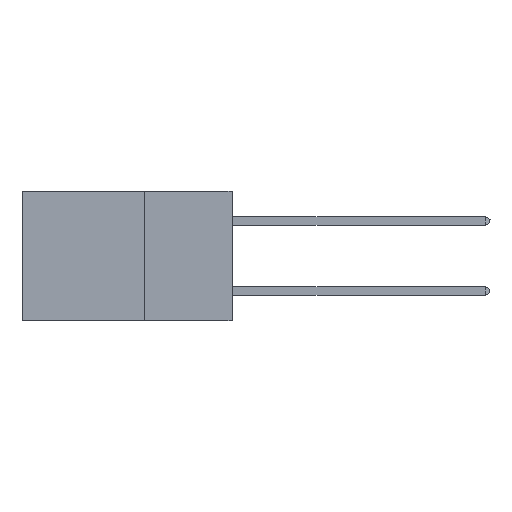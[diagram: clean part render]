
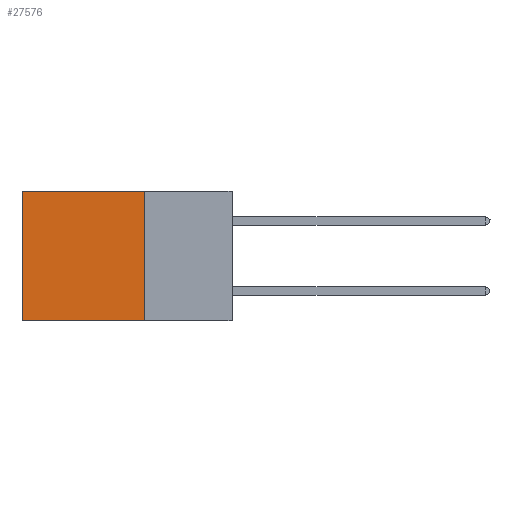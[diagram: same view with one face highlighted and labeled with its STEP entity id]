
A CAD part, left-side view. The second image highlights one B-rep face of the part: STEP entity #27576.
In plain terms, the highlighted planar face has unit normal (-1, 0, 0).
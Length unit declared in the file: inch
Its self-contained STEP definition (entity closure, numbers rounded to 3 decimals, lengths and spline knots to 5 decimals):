
#475 = ORIENTED_EDGE ( 'NONE', *, *, #20749, .F. ) ;
#2048 = VERTEX_POINT ( 'NONE', #22306 ) ;
#2935 = FACE_OUTER_BOUND ( 'NONE', #39956, .T. ) ;
#2964 = ORIENTED_EDGE ( 'NONE', *, *, #19915, .T. ) ;
#4848 = CARTESIAN_POINT ( 'NONE',  ( 0.2875, 0.25, -0.37 ) ) ;
#4908 = CARTESIAN_POINT ( 'NONE',  ( 0.2875, 0.25, 0. ) ) ;
#5237 = DIRECTION ( 'NONE',  ( 0., 0., -1. ) ) ;
#6970 = ORIENTED_EDGE ( 'NONE', *, *, #25599, .F. ) ;
#7284 = CARTESIAN_POINT ( 'NONE',  ( 0.2875, 0.25, 0. ) ) ;
#7676 = DIRECTION ( 'NONE',  ( 0., 1., 0. ) ) ;
#8285 = LINE ( 'NONE', #22041, #31286 ) ;
#8759 = LINE ( 'NONE', #9410, #9766 ) ;
#9410 = CARTESIAN_POINT ( 'NONE',  ( 0.2875, 0.25, 0. ) ) ;
#9766 = VECTOR ( 'NONE', #35423, 39.37008 ) ;
#9790 = VERTEX_POINT ( 'NONE', #36694 ) ;
#11019 = LINE ( 'NONE', #4908, #34777 ) ;
#15156 = VERTEX_POINT ( 'NONE', #33258 ) ;
#17466 = ORIENTED_EDGE ( 'NONE', *, *, #27463, .T. ) ;
#18236 = AXIS2_PLACEMENT_3D ( 'NONE', #39439, #33085, #42938 ) ;
#19915 = EDGE_CURVE ( 'NONE', #2048, #9790, #8285, .T. ) ;
#20749 = EDGE_CURVE ( 'NONE', #15156, #9790, #24489, .T. ) ;
#22041 = CARTESIAN_POINT ( 'NONE',  ( 0.2875, 0.6, 0. ) ) ;
#22306 = CARTESIAN_POINT ( 'NONE',  ( 0.2875, 0.6, 0. ) ) ;
#24489 = LINE ( 'NONE', #4848, #31104 ) ;
#25599 = EDGE_CURVE ( 'NONE', #35678, #15156, #8759, .T. ) ;
#27463 = EDGE_CURVE ( 'NONE', #35678, #2048, #11019, .T. ) ;
#27576 = ADVANCED_FACE ( 'NONE', ( #2935 ), #29587, .F. ) ;
#29587 = PLANE ( 'NONE',  #18236 ) ;
#30899 = DIRECTION ( 'NONE',  ( 0., 1., 0. ) ) ;
#31104 = VECTOR ( 'NONE', #7676, 39.37008 ) ;
#31286 = VECTOR ( 'NONE', #5237, 39.37008 ) ;
#33085 = DIRECTION ( 'NONE',  ( 1., 0., 0. ) ) ;
#33258 = CARTESIAN_POINT ( 'NONE',  ( 0.2875, 0.25, -0.37 ) ) ;
#34777 = VECTOR ( 'NONE', #30899, 39.37008 ) ;
#35423 = DIRECTION ( 'NONE',  ( 0., 0., -1. ) ) ;
#35678 = VERTEX_POINT ( 'NONE', #7284 ) ;
#36694 = CARTESIAN_POINT ( 'NONE',  ( 0.2875, 0.6, -0.37 ) ) ;
#39439 = CARTESIAN_POINT ( 'NONE',  ( 0.2875, 0.25, 0. ) ) ;
#39956 = EDGE_LOOP ( 'NONE', ( #2964, #475, #6970, #17466 ) ) ;
#42938 = DIRECTION ( 'NONE',  ( 0., 0., -1. ) ) ;
